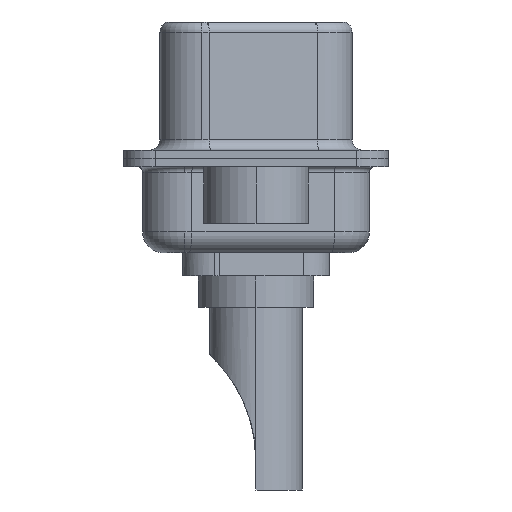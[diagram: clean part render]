
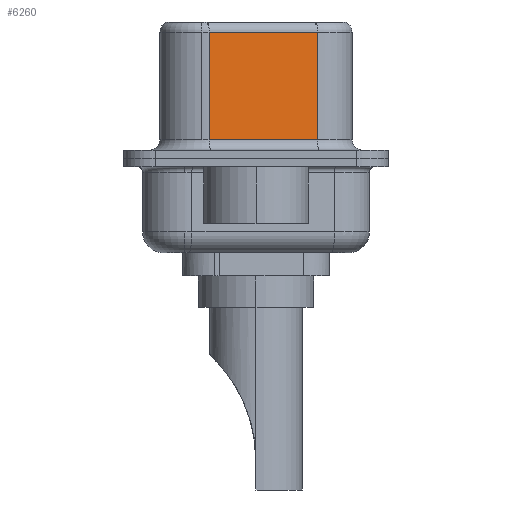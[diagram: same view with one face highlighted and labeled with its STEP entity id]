
A CAD part, left-side view. The second image highlights one B-rep face of the part: STEP entity #6260.
In plain terms, the highlighted planar face has unit normal (-0.985, -0.174, 0).
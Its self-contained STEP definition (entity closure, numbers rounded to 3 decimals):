
#146 = CARTESIAN_POINT ( 'NONE',  ( 3.67, 2.233, 0.9 ) ) ;
#185 = EDGE_CURVE ( 'NONE', #10592, #18616, #11843, .T. ) ;
#2361 = CARTESIAN_POINT ( 'NONE',  ( 3.67, 2.233, 6.52 ) ) ;
#2368 = VECTOR ( 'NONE', #9903, 1000. ) ;
#2743 = LINE ( 'NONE', #4956, #20532 ) ;
#3021 = VECTOR ( 'NONE', #9795, 1000. ) ;
#4733 = DIRECTION ( 'NONE',  ( -0.174, 0.985, 0. ) ) ;
#4956 = CARTESIAN_POINT ( 'NONE',  ( 4.58, -2.927, 0.9 ) ) ;
#6260 = ADVANCED_FACE ( 'NONE', ( #8197 ), #13588, .F. ) ;
#7986 = CARTESIAN_POINT ( 'NONE',  ( 4.58, -2.927, 6.02 ) ) ;
#8197 = FACE_OUTER_BOUND ( 'NONE', #22170, .T. ) ;
#8572 = LINE ( 'NONE', #15722, #17425 ) ;
#8709 = ORIENTED_EDGE ( 'NONE', *, *, #185, .T. ) ;
#9795 = DIRECTION ( 'NONE',  ( -0.174, 0.985, 0. ) ) ;
#9903 = DIRECTION ( 'NONE',  ( 0., 0., -1. ) ) ;
#10439 = ORIENTED_EDGE ( 'NONE', *, *, #13240, .T. ) ;
#10592 = VERTEX_POINT ( 'NONE', #16011 ) ;
#11843 = LINE ( 'NONE', #2361, #2368 ) ;
#12701 = EDGE_CURVE ( 'NONE', #18616, #19829, #2743, .T. ) ;
#13240 = EDGE_CURVE ( 'NONE', #20692, #10592, #21934, .T. ) ;
#13515 = CARTESIAN_POINT ( 'NONE',  ( 4.58, -2.927, 6.52 ) ) ;
#13588 = PLANE ( 'NONE',  #22242 ) ;
#13891 = ORIENTED_EDGE ( 'NONE', *, *, #12701, .T. ) ;
#15375 = DIRECTION ( 'NONE',  ( 0.985, 0.174, 0. ) ) ;
#15722 = CARTESIAN_POINT ( 'NONE',  ( 4.58, -2.927, 6.52 ) ) ;
#16011 = CARTESIAN_POINT ( 'NONE',  ( 3.67, 2.233, 6.02 ) ) ;
#16963 = CARTESIAN_POINT ( 'NONE',  ( 4.58, -2.927, 0.9 ) ) ;
#17425 = VECTOR ( 'NONE', #21005, 1000. ) ;
#18616 = VERTEX_POINT ( 'NONE', #146 ) ;
#19829 = VERTEX_POINT ( 'NONE', #16963 ) ;
#20532 = VECTOR ( 'NONE', #22747, 1000. ) ;
#20692 = VERTEX_POINT ( 'NONE', #21444 ) ;
#21005 = DIRECTION ( 'NONE',  ( 0., 0., -1. ) ) ;
#21444 = CARTESIAN_POINT ( 'NONE',  ( 4.58, -2.927, 6.02 ) ) ;
#21774 = EDGE_CURVE ( 'NONE', #20692, #19829, #8572, .T. ) ;
#21934 = LINE ( 'NONE', #7986, #3021 ) ;
#22047 = ORIENTED_EDGE ( 'NONE', *, *, #21774, .F. ) ;
#22170 = EDGE_LOOP ( 'NONE', ( #22047, #10439, #8709, #13891 ) ) ;
#22242 = AXIS2_PLACEMENT_3D ( 'NONE', #13515, #15375, #4733 ) ;
#22747 = DIRECTION ( 'NONE',  ( 0.174, -0.985, 0. ) ) ;
